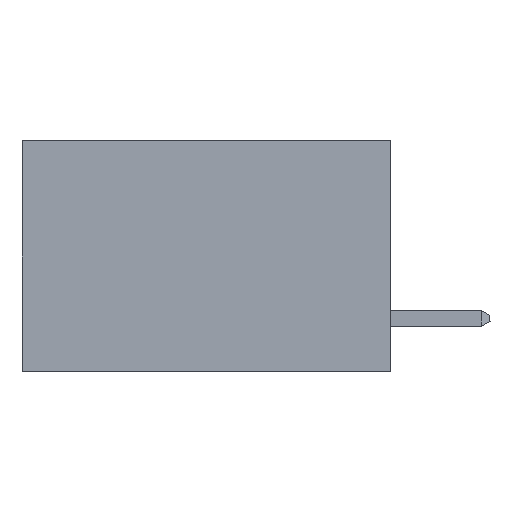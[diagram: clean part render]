
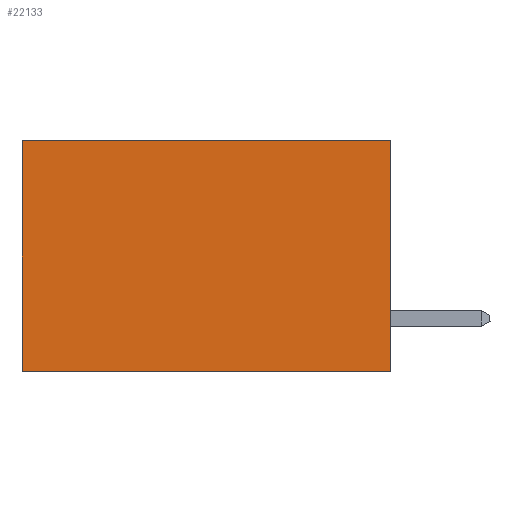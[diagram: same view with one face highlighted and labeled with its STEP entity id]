
A CAD part, left-side view. The second image highlights one B-rep face of the part: STEP entity #22133.
In plain terms, the highlighted planar face has unit normal (-1, 0, 0).
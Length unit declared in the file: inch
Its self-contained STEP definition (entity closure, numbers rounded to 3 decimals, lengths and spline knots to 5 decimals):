
#579 = CARTESIAN_POINT ( 'NONE',  ( 0.277, 0., -0.37 ) ) ;
#1901 = FACE_OUTER_BOUND ( 'NONE', #24996, .T. ) ;
#3252 = CARTESIAN_POINT ( 'NONE',  ( 0.277, 0.59, -0.37 ) ) ;
#3528 = CARTESIAN_POINT ( 'NONE',  ( 0.277, 0., 0. ) ) ;
#3659 = DIRECTION ( 'NONE',  ( 0., 0., -1. ) ) ;
#3983 = ORIENTED_EDGE ( 'NONE', *, *, #11286, .F. ) ;
#5403 = VECTOR ( 'NONE', #25277, 39.37008 ) ;
#6238 = ORIENTED_EDGE ( 'NONE', *, *, #18506, .T. ) ;
#6661 = VERTEX_POINT ( 'NONE', #3528 ) ;
#6845 = AXIS2_PLACEMENT_3D ( 'NONE', #7638, #15674, #3659 ) ;
#7638 = CARTESIAN_POINT ( 'NONE',  ( 0.277, 0., -0.37 ) ) ;
#7999 = DIRECTION ( 'NONE',  ( 0., 1., 0. ) ) ;
#8699 = VERTEX_POINT ( 'NONE', #3252 ) ;
#9395 = VECTOR ( 'NONE', #17618, 39.37008 ) ;
#10636 = LINE ( 'NONE', #25346, #9395 ) ;
#10970 = VECTOR ( 'NONE', #7999, 39.37008 ) ;
#11286 = EDGE_CURVE ( 'NONE', #21822, #8699, #16307, .T. ) ;
#11996 = LINE ( 'NONE', #23323, #5403 ) ;
#13648 = PLANE ( 'NONE',  #6845 ) ;
#13860 = CARTESIAN_POINT ( 'NONE',  ( 0.277, 0., -0.37 ) ) ;
#14725 = EDGE_CURVE ( 'NONE', #6661, #21822, #25722, .T. ) ;
#15674 = DIRECTION ( 'NONE',  ( 1., 0., 0. ) ) ;
#15956 = CARTESIAN_POINT ( 'NONE',  ( 0.277, 0., -0.37 ) ) ;
#16307 = LINE ( 'NONE', #15956, #10970 ) ;
#17000 = CARTESIAN_POINT ( 'NONE',  ( 0.277, 0.59, 0. ) ) ;
#17485 = ORIENTED_EDGE ( 'NONE', *, *, #23457, .T. ) ;
#17618 = DIRECTION ( 'NONE',  ( 0., 1., 0. ) ) ;
#17881 = DIRECTION ( 'NONE',  ( 0., 0., -1. ) ) ;
#18506 = EDGE_CURVE ( 'NONE', #23275, #8699, #11996, .T. ) ;
#20576 = VECTOR ( 'NONE', #17881, 39.37008 ) ;
#21822 = VERTEX_POINT ( 'NONE', #579 ) ;
#22133 = ADVANCED_FACE ( 'NONE', ( #1901 ), #13648, .F. ) ;
#22359 = ORIENTED_EDGE ( 'NONE', *, *, #14725, .F. ) ;
#23275 = VERTEX_POINT ( 'NONE', #17000 ) ;
#23323 = CARTESIAN_POINT ( 'NONE',  ( 0.277, 0.59, -0.37 ) ) ;
#23457 = EDGE_CURVE ( 'NONE', #6661, #23275, #10636, .T. ) ;
#24996 = EDGE_LOOP ( 'NONE', ( #6238, #3983, #22359, #17485 ) ) ;
#25277 = DIRECTION ( 'NONE',  ( 0., 0., -1. ) ) ;
#25346 = CARTESIAN_POINT ( 'NONE',  ( 0.277, 0., 0. ) ) ;
#25722 = LINE ( 'NONE', #13860, #20576 ) ;
